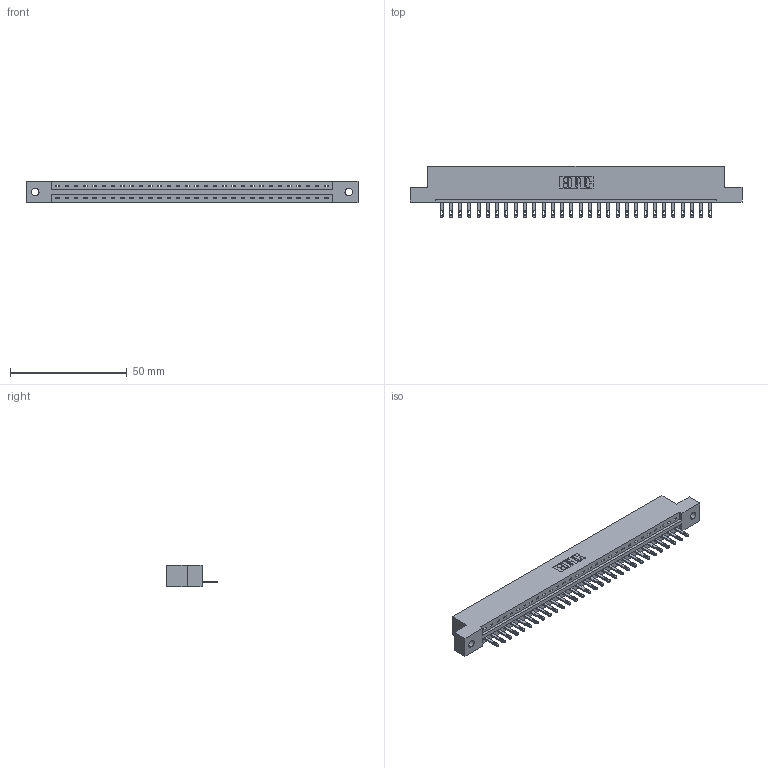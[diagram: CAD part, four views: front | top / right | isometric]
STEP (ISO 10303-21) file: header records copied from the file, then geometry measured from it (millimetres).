
FILE_DESCRIPTION (( 'STEP AP203' ), '1' );
FILE_NAME ('887-030-500-102.STEP', '2020-09-20T20:28:49', ( '' ), ( '' ), 'SwSTEP 2.0', 'SolidWorks 2020', '' );
FILE_SCHEMA (( 'CONFIG_CONTROL_DESIGN' ));
Length unit declared in the file: inch
Products named in the file (3): 837 Part_Flush Mounting Lugs - 0.128 Dia; 887-030-500-102; 345-292-001_345-293-100
Assembly tree (31 placements, depth 2):
  887-030-500-102
    837 Part_Flush Mounting Lugs - 0.128 Dia
    345-292-001_345-293-100  x30
Bounding box: 141.88 x 21.85 x 9.4 mm (x, y, z)
Volume: 14578.2 mm3; surface area: 14798 mm2
Topology: 31 solids, 31 shells, 1854 faces, 5711 edges, 3806 vertices
Faces by surface type: plane 1270, cylinder 584
Entity records: 23785 total; most frequent: CARTESIAN_POINT 4148, ORIENTED_EDGE 4114, DIRECTION 3517, EDGE_CURVE 2057, LINE 1925, VECTOR 1925, VERTEX_POINT 1370, AXIS2_PLACEMENT_3D 796
